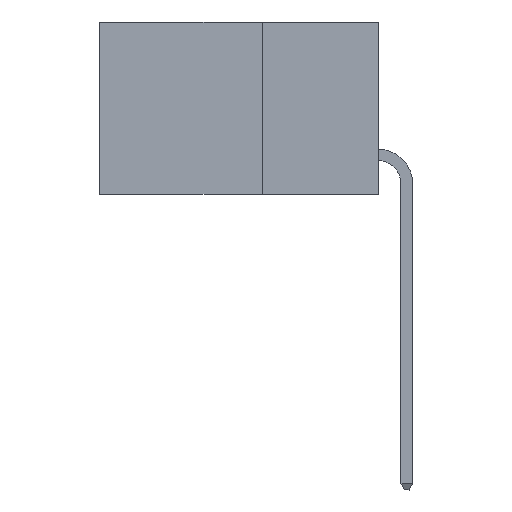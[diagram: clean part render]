
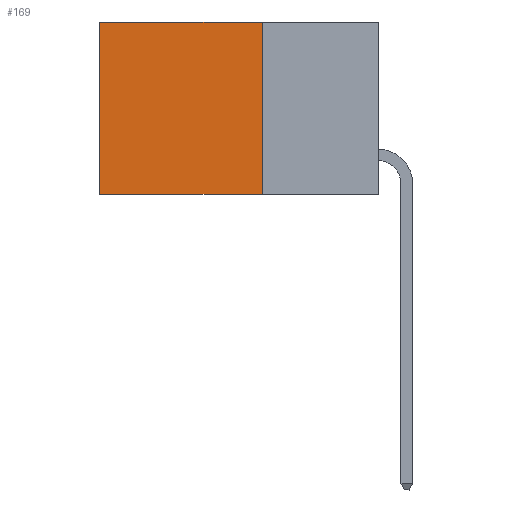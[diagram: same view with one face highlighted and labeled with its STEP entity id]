
A CAD part, left-side view. The second image highlights one B-rep face of the part: STEP entity #169.
In plain terms, the highlighted planar face has unit normal (-1, 0, 0).
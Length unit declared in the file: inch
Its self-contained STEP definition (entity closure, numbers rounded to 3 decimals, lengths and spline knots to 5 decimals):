
#169 = ADVANCED_FACE ( 'NONE', ( #12680 ), #638, .F. ) ;
#304 = LINE ( 'NONE', #14946, #5965 ) ;
#419 = CARTESIAN_POINT ( 'NONE',  ( 0.2615, 0.6, 0. ) ) ;
#635 = EDGE_LOOP ( 'NONE', ( #5483, #6770, #13998, #3567 ) ) ;
#638 = PLANE ( 'NONE',  #7129 ) ;
#1580 = VECTOR ( 'NONE', #4341, 39.37008 ) ;
#1985 = CARTESIAN_POINT ( 'NONE',  ( 0.2615, 0.25, -0.37 ) ) ;
#2225 = LINE ( 'NONE', #1985, #3946 ) ;
#2952 = EDGE_CURVE ( 'NONE', #14905, #3853, #15161, .T. ) ;
#3567 = ORIENTED_EDGE ( 'NONE', *, *, #8170, .T. ) ;
#3853 = VERTEX_POINT ( 'NONE', #9421 ) ;
#3946 = VECTOR ( 'NONE', #4557, 39.37008 ) ;
#4341 = DIRECTION ( 'NONE',  ( 0., 0., -1. ) ) ;
#4557 = DIRECTION ( 'NONE',  ( 0., 1., 0. ) ) ;
#4757 = DIRECTION ( 'NONE',  ( 0., 1., 0. ) ) ;
#5483 = ORIENTED_EDGE ( 'NONE', *, *, #2952, .T. ) ;
#5577 = VERTEX_POINT ( 'NONE', #8937 ) ;
#5965 = VECTOR ( 'NONE', #12500, 39.37008 ) ;
#6770 = ORIENTED_EDGE ( 'NONE', *, *, #13417, .F. ) ;
#7129 = AXIS2_PLACEMENT_3D ( 'NONE', #11497, #10377, #8041 ) ;
#8041 = DIRECTION ( 'NONE',  ( 0., 0., -1. ) ) ;
#8170 = EDGE_CURVE ( 'NONE', #5577, #14905, #14469, .T. ) ;
#8937 = CARTESIAN_POINT ( 'NONE',  ( 0.2615, 0.25, 0. ) ) ;
#9421 = CARTESIAN_POINT ( 'NONE',  ( 0.2615, 0.6, -0.37 ) ) ;
#10159 = VERTEX_POINT ( 'NONE', #14951 ) ;
#10297 = VECTOR ( 'NONE', #4757, 39.37008 ) ;
#10377 = DIRECTION ( 'NONE',  ( 1., 0., 0. ) ) ;
#10745 = CARTESIAN_POINT ( 'NONE',  ( 0.2615, 0.25, 0. ) ) ;
#11497 = CARTESIAN_POINT ( 'NONE',  ( 0.2615, 0.25, -0.37 ) ) ;
#11600 = CARTESIAN_POINT ( 'NONE',  ( 0.2615, 0.6, -0.37 ) ) ;
#12500 = DIRECTION ( 'NONE',  ( 0., 0., -1. ) ) ;
#12680 = FACE_OUTER_BOUND ( 'NONE', #635, .T. ) ;
#12913 = EDGE_CURVE ( 'NONE', #5577, #10159, #304, .T. ) ;
#13417 = EDGE_CURVE ( 'NONE', #10159, #3853, #2225, .T. ) ;
#13998 = ORIENTED_EDGE ( 'NONE', *, *, #12913, .F. ) ;
#14469 = LINE ( 'NONE', #10745, #10297 ) ;
#14905 = VERTEX_POINT ( 'NONE', #419 ) ;
#14946 = CARTESIAN_POINT ( 'NONE',  ( 0.2615, 0.25, -0.37 ) ) ;
#14951 = CARTESIAN_POINT ( 'NONE',  ( 0.2615, 0.25, -0.37 ) ) ;
#15161 = LINE ( 'NONE', #11600, #1580 ) ;
